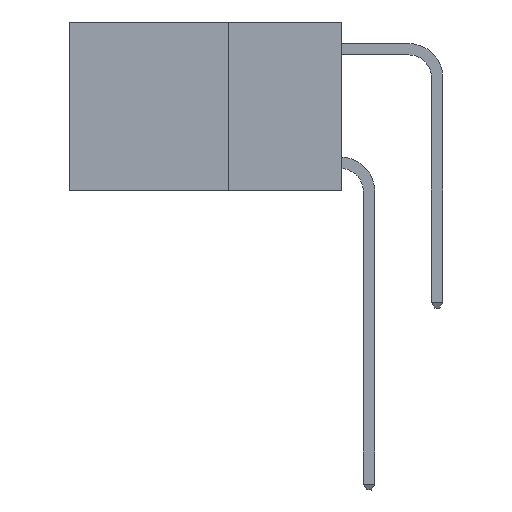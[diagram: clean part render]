
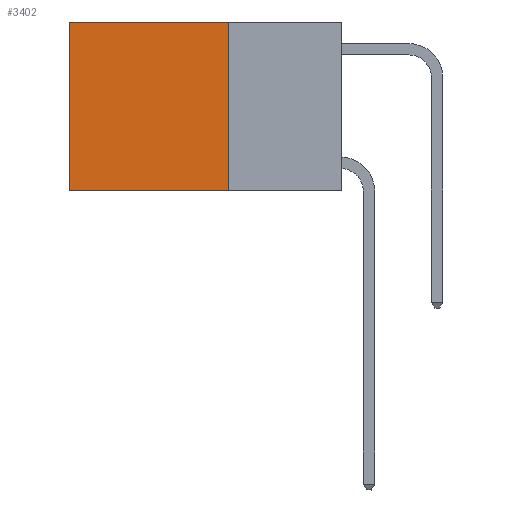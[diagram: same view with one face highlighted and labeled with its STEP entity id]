
A CAD part, left-side view. The second image highlights one B-rep face of the part: STEP entity #3402.
In plain terms, the highlighted planar face has unit normal (-1, 0, 0).
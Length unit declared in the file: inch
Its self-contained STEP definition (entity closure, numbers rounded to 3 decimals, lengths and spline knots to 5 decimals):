
#256 = DIRECTION ( 'NONE',  ( 0., 0., -1. ) ) ;
#469 = LINE ( 'NONE', #2494, #5904 ) ;
#672 = LINE ( 'NONE', #6247, #5438 ) ;
#1259 = ORIENTED_EDGE ( 'NONE', *, *, #3942, .T. ) ;
#1276 = CARTESIAN_POINT ( 'NONE',  ( 0.2625, 0.6, -0.37 ) ) ;
#1975 = VECTOR ( 'NONE', #256, 39.37008 ) ;
#2494 = CARTESIAN_POINT ( 'NONE',  ( 0.2625, 0.25, 0. ) ) ;
#2959 = CARTESIAN_POINT ( 'NONE',  ( 0.2625, 0.25, -0.37 ) ) ;
#3013 = AXIS2_PLACEMENT_3D ( 'NONE', #4217, #12415, #6372 ) ;
#3343 = VERTEX_POINT ( 'NONE', #5263 ) ;
#3402 = ADVANCED_FACE ( 'NONE', ( #11323 ), #5357, .F. ) ;
#3480 = CARTESIAN_POINT ( 'NONE',  ( 0.2625, 0.25, 0. ) ) ;
#3942 = EDGE_CURVE ( 'NONE', #3343, #4041, #12970, .T. ) ;
#4041 = VERTEX_POINT ( 'NONE', #1276 ) ;
#4217 = CARTESIAN_POINT ( 'NONE',  ( 0.2625, 0.25, 0. ) ) ;
#4382 = EDGE_CURVE ( 'NONE', #7943, #4041, #672, .T. ) ;
#4467 = ORIENTED_EDGE ( 'NONE', *, *, #6885, .F. ) ;
#4504 = EDGE_CURVE ( 'NONE', #10886, #3343, #469, .T. ) ;
#4829 = LINE ( 'NONE', #8685, #1975 ) ;
#5263 = CARTESIAN_POINT ( 'NONE',  ( 0.2625, 0.6, 0. ) ) ;
#5357 = PLANE ( 'NONE',  #3013 ) ;
#5438 = VECTOR ( 'NONE', #7256, 39.37008 ) ;
#5904 = VECTOR ( 'NONE', #10803, 39.37008 ) ;
#6207 = ORIENTED_EDGE ( 'NONE', *, *, #4504, .T. ) ;
#6247 = CARTESIAN_POINT ( 'NONE',  ( 0.2625, 0.25, -0.37 ) ) ;
#6352 = DIRECTION ( 'NONE',  ( 0., 0., -1. ) ) ;
#6372 = DIRECTION ( 'NONE',  ( 0., 0., -1. ) ) ;
#6885 = EDGE_CURVE ( 'NONE', #10886, #7943, #4829, .T. ) ;
#7256 = DIRECTION ( 'NONE',  ( 0., 1., 0. ) ) ;
#7943 = VERTEX_POINT ( 'NONE', #2959 ) ;
#8685 = CARTESIAN_POINT ( 'NONE',  ( 0.2625, 0.25, 0. ) ) ;
#9614 = ORIENTED_EDGE ( 'NONE', *, *, #4382, .F. ) ;
#9737 = VECTOR ( 'NONE', #6352, 39.37008 ) ;
#10803 = DIRECTION ( 'NONE',  ( 0., 1., 0. ) ) ;
#10886 = VERTEX_POINT ( 'NONE', #3480 ) ;
#11323 = FACE_OUTER_BOUND ( 'NONE', #12303, .T. ) ;
#12303 = EDGE_LOOP ( 'NONE', ( #1259, #9614, #4467, #6207 ) ) ;
#12361 = CARTESIAN_POINT ( 'NONE',  ( 0.2625, 0.6, 0. ) ) ;
#12415 = DIRECTION ( 'NONE',  ( 1., 0., 0. ) ) ;
#12970 = LINE ( 'NONE', #12361, #9737 ) ;
